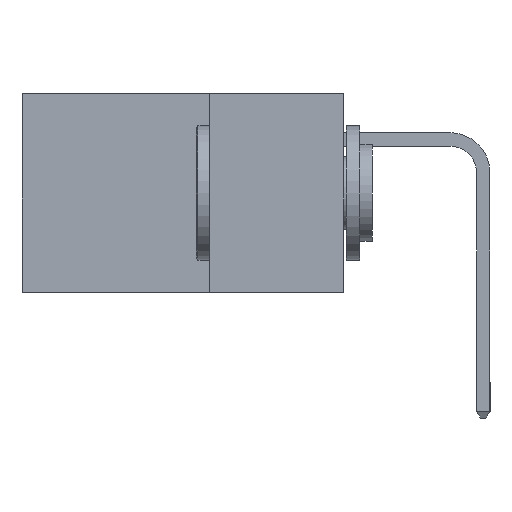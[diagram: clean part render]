
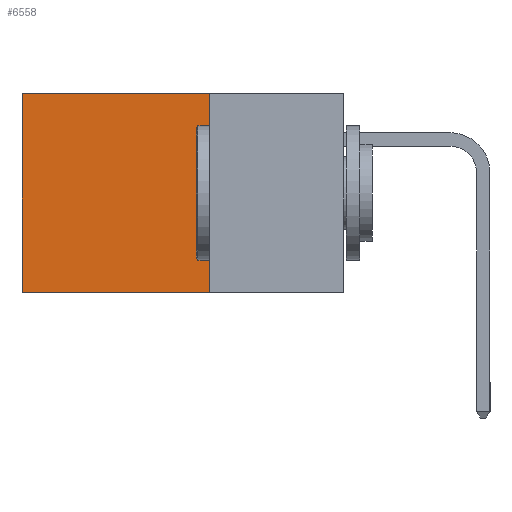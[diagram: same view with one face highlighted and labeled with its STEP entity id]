
A CAD part, left-side view. The second image highlights one B-rep face of the part: STEP entity #6558.
In plain terms, the highlighted planar face has unit normal (-1, 0, 0).
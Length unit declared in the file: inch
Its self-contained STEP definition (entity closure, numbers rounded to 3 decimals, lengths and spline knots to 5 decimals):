
#97 = ORIENTED_EDGE ( 'NONE', *, *, #13318, .T. ) ;
#855 = VERTEX_POINT ( 'NONE', #7541 ) ;
#1833 = LINE ( 'NONE', #9123, #11883 ) ;
#2119 = LINE ( 'NONE', #2335, #12150 ) ;
#2237 = EDGE_CURVE ( 'NONE', #13581, #7712, #10519, .T. ) ;
#2335 = CARTESIAN_POINT ( 'NONE',  ( 0.298, 0.6, 0. ) ) ;
#3908 = VECTOR ( 'NONE', #16473, 39.37008 ) ;
#5444 = ORIENTED_EDGE ( 'NONE', *, *, #8656, .T. ) ;
#5912 = VERTEX_POINT ( 'NONE', #8105 ) ;
#6291 = ORIENTED_EDGE ( 'NONE', *, *, #11793, .F. ) ;
#6464 = AXIS2_PLACEMENT_3D ( 'NONE', #12106, #12032, #11965 ) ;
#6558 = ADVANCED_FACE ( 'NONE', ( #9605 ), #12221, .F. ) ;
#7541 = CARTESIAN_POINT ( 'NONE',  ( 0.298, 0.6, 0. ) ) ;
#7712 = VERTEX_POINT ( 'NONE', #10966 ) ;
#7881 = DIRECTION ( 'NONE',  ( 0., 0., -1. ) ) ;
#8105 = CARTESIAN_POINT ( 'NONE',  ( 0.298, 0.25, 0. ) ) ;
#8656 = EDGE_CURVE ( 'NONE', #855, #7712, #2119, .T. ) ;
#9123 = CARTESIAN_POINT ( 'NONE',  ( 0.298, 0.25, 0. ) ) ;
#9605 = FACE_OUTER_BOUND ( 'NONE', #16205, .T. ) ;
#9661 = CARTESIAN_POINT ( 'NONE',  ( 0.298, 0.25, -0.37 ) ) ;
#9954 = DIRECTION ( 'NONE',  ( 0., 1., 0. ) ) ;
#10519 = LINE ( 'NONE', #9661, #13483 ) ;
#10646 = ORIENTED_EDGE ( 'NONE', *, *, #2237, .F. ) ;
#10966 = CARTESIAN_POINT ( 'NONE',  ( 0.298, 0.6, -0.37 ) ) ;
#11793 = EDGE_CURVE ( 'NONE', #5912, #13581, #1833, .T. ) ;
#11883 = VECTOR ( 'NONE', #7881, 39.37008 ) ;
#11965 = DIRECTION ( 'NONE',  ( 0., 0., -1. ) ) ;
#12032 = DIRECTION ( 'NONE',  ( 1., 0., 0. ) ) ;
#12106 = CARTESIAN_POINT ( 'NONE',  ( 0.298, 0.25, 0. ) ) ;
#12150 = VECTOR ( 'NONE', #13926, 39.37008 ) ;
#12221 = PLANE ( 'NONE',  #6464 ) ;
#13318 = EDGE_CURVE ( 'NONE', #5912, #855, #14141, .T. ) ;
#13394 = CARTESIAN_POINT ( 'NONE',  ( 0.298, 0.25, -0.37 ) ) ;
#13483 = VECTOR ( 'NONE', #9954, 39.37008 ) ;
#13581 = VERTEX_POINT ( 'NONE', #13394 ) ;
#13926 = DIRECTION ( 'NONE',  ( 0., 0., -1. ) ) ;
#14075 = CARTESIAN_POINT ( 'NONE',  ( 0.298, 0.25, 0. ) ) ;
#14141 = LINE ( 'NONE', #14075, #3908 ) ;
#16205 = EDGE_LOOP ( 'NONE', ( #5444, #10646, #6291, #97 ) ) ;
#16473 = DIRECTION ( 'NONE',  ( 0., 1., 0. ) ) ;
